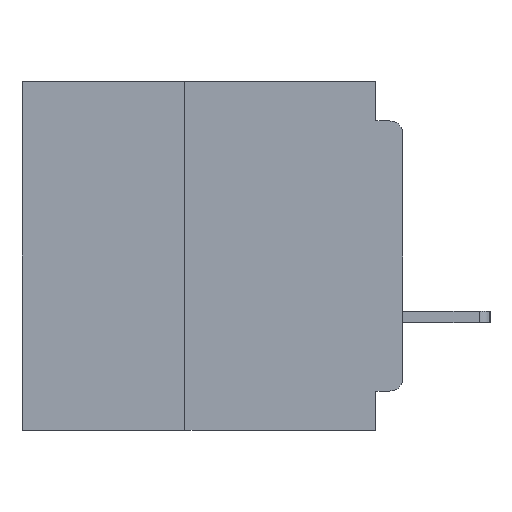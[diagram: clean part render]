
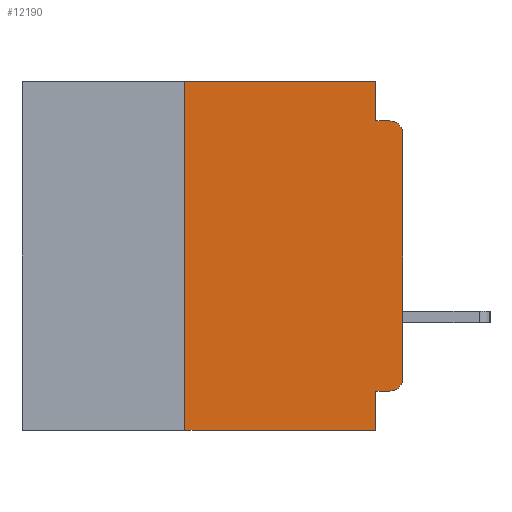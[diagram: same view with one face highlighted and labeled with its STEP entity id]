
A CAD part, left-side view. The second image highlights one B-rep face of the part: STEP entity #12190.
In plain terms, the highlighted planar face has unit normal (-1, 0, 0).
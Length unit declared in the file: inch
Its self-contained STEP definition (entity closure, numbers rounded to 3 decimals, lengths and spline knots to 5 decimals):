
#1024 = DIRECTION ( 'NONE',  ( 0., 0., 1. ) ) ;
#1780 = ORIENTED_EDGE ( 'NONE', *, *, #16107, .T. ) ;
#1989 = EDGE_CURVE ( 'NONE', #16276, #15514, #10104, .T. ) ;
#2126 = DIRECTION ( 'NONE',  ( 0., 0., -1. ) ) ;
#2932 = EDGE_CURVE ( 'NONE', #9208, #16276, #19423, .T. ) ;
#3079 = ORIENTED_EDGE ( 'NONE', *, *, #32618, .T. ) ;
#3225 = CARTESIAN_POINT ( 'NONE',  ( 0., 0.031, 0. ) ) ;
#4068 = ORIENTED_EDGE ( 'NONE', *, *, #34736, .T. ) ;
#4883 = DIRECTION ( 'NONE',  ( 0., 0., 1. ) ) ;
#6732 = ORIENTED_EDGE ( 'NONE', *, *, #19267, .F. ) ;
#8090 = CARTESIAN_POINT ( 'NONE',  ( 0., 0.015, -0.045 ) ) ;
#8236 = FACE_OUTER_BOUND ( 'NONE', #32101, .T. ) ;
#8343 = CARTESIAN_POINT ( 'NONE',  ( 0., 0.25, -0.4 ) ) ;
#8679 = CARTESIAN_POINT ( 'NONE',  ( 0., 0.031, -0.4 ) ) ;
#9208 = VERTEX_POINT ( 'NONE', #21898 ) ;
#10104 = LINE ( 'NONE', #8679, #17839 ) ;
#11423 = VECTOR ( 'NONE', #25839, 39.37008 ) ;
#11497 = DIRECTION ( 'NONE',  ( 0., 0., -1. ) ) ;
#11811 = EDGE_CURVE ( 'NONE', #31311, #32200, #21904, .T. ) ;
#12190 = ADVANCED_FACE ( 'NONE', ( #8236 ), #23067, .F. ) ;
#13192 = CARTESIAN_POINT ( 'NONE',  ( 0., 0., -0.355 ) ) ;
#13544 = ORIENTED_EDGE ( 'NONE', *, *, #26855, .F. ) ;
#14096 = CARTESIAN_POINT ( 'NONE',  ( 0., 0.437, 0. ) ) ;
#14188 = CARTESIAN_POINT ( 'NONE',  ( 0., 0.015, -0.34 ) ) ;
#14190 = VECTOR ( 'NONE', #1024, 39.37008 ) ;
#14222 = DIRECTION ( 'NONE',  ( 0., -1., 0. ) ) ;
#14447 = VECTOR ( 'NONE', #14222, 39.37008 ) ;
#15514 = VERTEX_POINT ( 'NONE', #18472 ) ;
#16100 = VERTEX_POINT ( 'NONE', #8343 ) ;
#16107 = EDGE_CURVE ( 'NONE', #16100, #15514, #34470, .T. ) ;
#16276 = VERTEX_POINT ( 'NONE', #35178 ) ;
#16311 = AXIS2_PLACEMENT_3D ( 'NONE', #36647, #19477, #2126 ) ;
#16726 = VECTOR ( 'NONE', #4883, 39.37008 ) ;
#16822 = CARTESIAN_POINT ( 'NONE',  ( 0., 0.25, 0. ) ) ;
#17099 = DIRECTION ( 'NONE',  ( 0., 0., -1. ) ) ;
#17218 = ORIENTED_EDGE ( 'NONE', *, *, #1989, .F. ) ;
#17234 = CARTESIAN_POINT ( 'NONE',  ( 0., 0.437, 0. ) ) ;
#17839 = VECTOR ( 'NONE', #23178, 39.37008 ) ;
#17871 = VERTEX_POINT ( 'NONE', #8090 ) ;
#18040 = LINE ( 'NONE', #31086, #31608 ) ;
#18138 = AXIS2_PLACEMENT_3D ( 'NONE', #17234, #28853, #11497 ) ;
#18472 = CARTESIAN_POINT ( 'NONE',  ( 0., 0.031, -0.4 ) ) ;
#18504 = ORIENTED_EDGE ( 'NONE', *, *, #35221, .F. ) ;
#18506 = VECTOR ( 'NONE', #21843, 39.37008 ) ;
#19142 = CIRCLE ( 'NONE', #16311, 0.015 ) ;
#19266 = CARTESIAN_POINT ( 'NONE',  ( 0., 0.031, -0.045 ) ) ;
#19267 = EDGE_CURVE ( 'NONE', #16100, #35265, #24406, .T. ) ;
#19423 = LINE ( 'NONE', #13192, #18506 ) ;
#19441 = DIRECTION ( 'NONE',  ( 0., 0., -1. ) ) ;
#19477 = DIRECTION ( 'NONE',  ( -1., 0., 0. ) ) ;
#20805 = CIRCLE ( 'NONE', #32533, 0.015 ) ;
#21351 = CARTESIAN_POINT ( 'NONE',  ( 0., 0., -0.34 ) ) ;
#21467 = VECTOR ( 'NONE', #19441, 39.37008 ) ;
#21843 = DIRECTION ( 'NONE',  ( 0., 1., 0. ) ) ;
#21898 = CARTESIAN_POINT ( 'NONE',  ( 0., 0.015, -0.355 ) ) ;
#21904 = LINE ( 'NONE', #35595, #14190 ) ;
#22166 = LINE ( 'NONE', #14096, #14447 ) ;
#22528 = DIRECTION ( 'NONE',  ( 0., -1., 0. ) ) ;
#23067 = PLANE ( 'NONE',  #18138 ) ;
#23178 = DIRECTION ( 'NONE',  ( 0., 0., -1. ) ) ;
#24362 = EDGE_CURVE ( 'NONE', #37118, #25463, #36679, .T. ) ;
#24406 = LINE ( 'NONE', #33559, #16726 ) ;
#25463 = VERTEX_POINT ( 'NONE', #19266 ) ;
#25839 = DIRECTION ( 'NONE',  ( 0., -1., 0. ) ) ;
#26855 = EDGE_CURVE ( 'NONE', #35265, #37118, #22166, .T. ) ;
#28853 = DIRECTION ( 'NONE',  ( 1., 0., 0. ) ) ;
#31086 = CARTESIAN_POINT ( 'NONE',  ( 0., 0., -0.045 ) ) ;
#31311 = VERTEX_POINT ( 'NONE', #21351 ) ;
#31608 = VECTOR ( 'NONE', #22528, 39.37008 ) ;
#31761 = CARTESIAN_POINT ( 'NONE',  ( 0., 0., -0.06 ) ) ;
#32101 = EDGE_LOOP ( 'NONE', ( #36901, #3079, #18504, #35594, #13544, #6732, #1780, #17218, #34340, #4068 ) ) ;
#32200 = VERTEX_POINT ( 'NONE', #31761 ) ;
#32533 = AXIS2_PLACEMENT_3D ( 'NONE', #14188, #34342, #17099 ) ;
#32618 = EDGE_CURVE ( 'NONE', #32200, #17871, #19142, .T. ) ;
#33559 = CARTESIAN_POINT ( 'NONE',  ( 0., 0.25, -0.4 ) ) ;
#33929 = CARTESIAN_POINT ( 'NONE',  ( 0., 0.031, 0. ) ) ;
#34340 = ORIENTED_EDGE ( 'NONE', *, *, #2932, .F. ) ;
#34342 = DIRECTION ( 'NONE',  ( -1., 0., 0. ) ) ;
#34353 = CARTESIAN_POINT ( 'NONE',  ( 0., 0.437, -0.4 ) ) ;
#34470 = LINE ( 'NONE', #34353, #11423 ) ;
#34736 = EDGE_CURVE ( 'NONE', #9208, #31311, #20805, .T. ) ;
#35178 = CARTESIAN_POINT ( 'NONE',  ( 0., 0.031, -0.355 ) ) ;
#35221 = EDGE_CURVE ( 'NONE', #25463, #17871, #18040, .T. ) ;
#35265 = VERTEX_POINT ( 'NONE', #16822 ) ;
#35594 = ORIENTED_EDGE ( 'NONE', *, *, #24362, .F. ) ;
#35595 = CARTESIAN_POINT ( 'NONE',  ( 0., 0., 0. ) ) ;
#36647 = CARTESIAN_POINT ( 'NONE',  ( 0., 0.015, -0.06 ) ) ;
#36679 = LINE ( 'NONE', #33929, #21467 ) ;
#36901 = ORIENTED_EDGE ( 'NONE', *, *, #11811, .T. ) ;
#37118 = VERTEX_POINT ( 'NONE', #3225 ) ;
